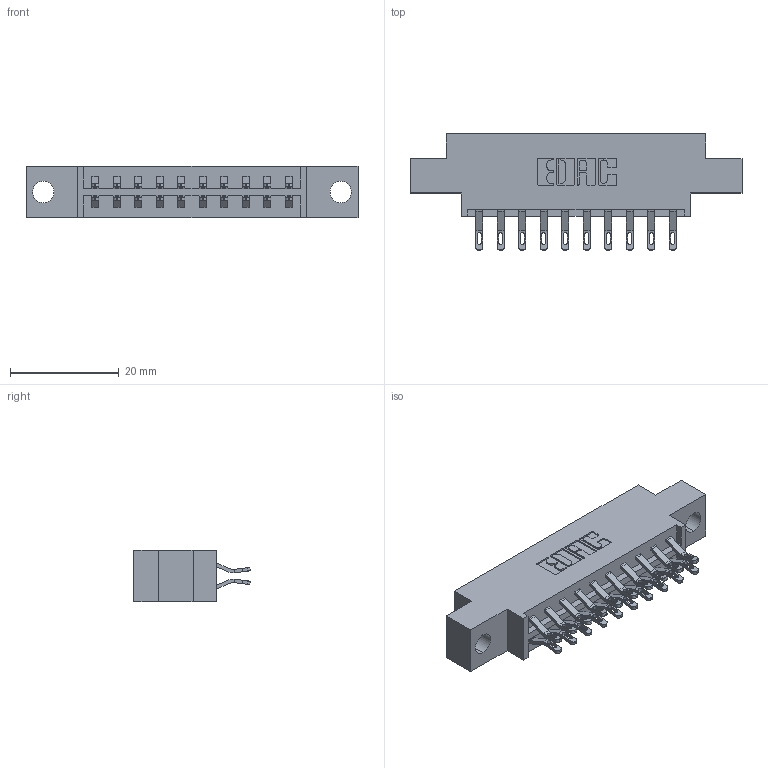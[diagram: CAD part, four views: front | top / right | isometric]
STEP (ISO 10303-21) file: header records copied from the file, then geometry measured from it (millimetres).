
FILE_DESCRIPTION (( 'STEP AP203' ), '1' );
FILE_NAME ('333-020-555-804.STEP', '2018-08-02T00:27:23', ( '' ), ( '' ), 'SwSTEP 2.0', 'SolidWorks 2016', '' );
FILE_SCHEMA (( 'CONFIG_CONTROL_DESIGN' ));
Length unit declared in the file: inch
Products named in the file (3): 333 Part_Offset - .156 Dia - TH; 345-292-001_555 Tail; 333-020-555-804
Assembly tree (21 placements, depth 2):
  333-020-555-804
    333 Part_Offset - .156 Dia - TH
    345-292-001_555 Tail  x20
Bounding box: 61.16 x 21.47 x 9.4 mm (x, y, z)
Volume: 5687.5 mm3; surface area: 6617.4 mm2
Topology: 21 solids, 21 shells, 1278 faces, 3983 edges, 2654 vertices
Faces by surface type: plane 754, cylinder 524
Entity records: 11033 total; most frequent: CARTESIAN_POINT 1904, ORIENTED_EDGE 1810, DIRECTION 1653, EDGE_CURVE 905, VECTOR 757, LINE 757, VERTEX_POINT 602, AXIS2_PLACEMENT_3D 448
